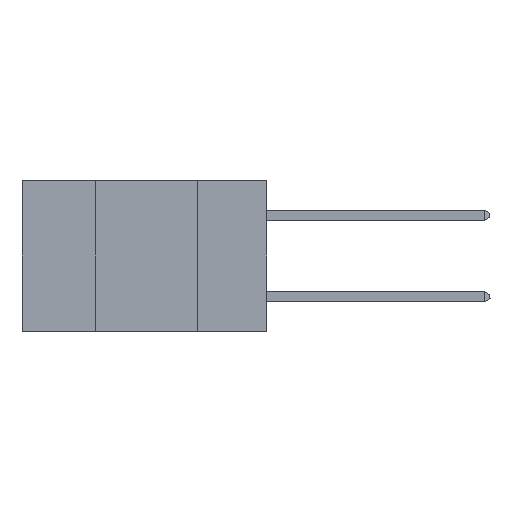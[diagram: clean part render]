
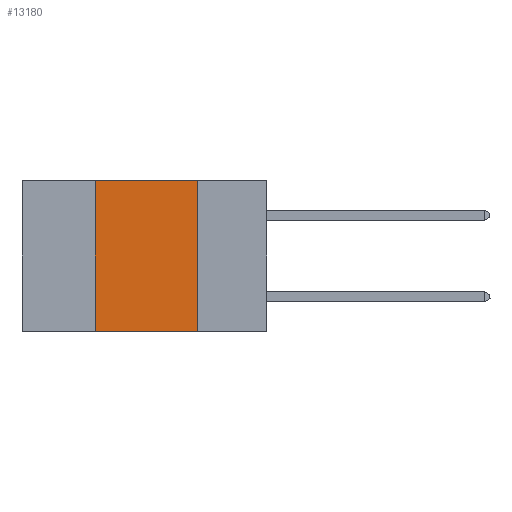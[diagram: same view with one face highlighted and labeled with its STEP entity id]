
A CAD part, left-side view. The second image highlights one B-rep face of the part: STEP entity #13180.
In plain terms, the highlighted planar face has unit normal (-1, 0, 0).
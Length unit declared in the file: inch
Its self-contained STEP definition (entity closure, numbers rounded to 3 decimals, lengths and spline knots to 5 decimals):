
#505 = EDGE_CURVE ( 'NONE', #16563, #8109, #4141, .T. ) ;
#512 = AXIS2_PLACEMENT_3D ( 'NONE', #13867, #15022, #13642 ) ;
#747 = PLANE ( 'NONE',  #512 ) ;
#1017 = EDGE_CURVE ( 'NONE', #11627, #1910, #9396, .T. ) ;
#1866 = ORIENTED_EDGE ( 'NONE', *, *, #1017, .F. ) ;
#1910 = VERTEX_POINT ( 'NONE', #3452 ) ;
#1997 = DIRECTION ( 'NONE',  ( 0., 0., 1. ) ) ;
#2954 = ORIENTED_EDGE ( 'NONE', *, *, #6083, .T. ) ;
#3342 = VECTOR ( 'NONE', #11138, 39.37008 ) ;
#3452 = CARTESIAN_POINT ( 'NONE',  ( 0., 0.17, -0.37 ) ) ;
#4040 = EDGE_LOOP ( 'NONE', ( #1866, #10951, #12915, #2954 ) ) ;
#4141 = LINE ( 'NONE', #8445, #13857 ) ;
#5557 = DIRECTION ( 'NONE',  ( 0., 0., -1. ) ) ;
#6083 = EDGE_CURVE ( 'NONE', #16563, #1910, #7611, .T. ) ;
#7055 = EDGE_CURVE ( 'NONE', #8109, #11627, #14868, .T. ) ;
#7611 = LINE ( 'NONE', #15401, #3342 ) ;
#8109 = VERTEX_POINT ( 'NONE', #9069 ) ;
#8445 = CARTESIAN_POINT ( 'NONE',  ( 0., 0.42, 0. ) ) ;
#9069 = CARTESIAN_POINT ( 'NONE',  ( 0., 0.42, 0. ) ) ;
#9396 = LINE ( 'NONE', #14796, #16338 ) ;
#9911 = FACE_OUTER_BOUND ( 'NONE', #4040, .T. ) ;
#10839 = CARTESIAN_POINT ( 'NONE',  ( 0., 0.17, 0. ) ) ;
#10951 = ORIENTED_EDGE ( 'NONE', *, *, #7055, .F. ) ;
#11138 = DIRECTION ( 'NONE',  ( 0., -1., 0. ) ) ;
#11627 = VERTEX_POINT ( 'NONE', #10839 ) ;
#12032 = DIRECTION ( 'NONE',  ( 0., -1., 0. ) ) ;
#12915 = ORIENTED_EDGE ( 'NONE', *, *, #505, .F. ) ;
#13180 = ADVANCED_FACE ( 'NONE', ( #9911 ), #747, .F. ) ;
#13642 = DIRECTION ( 'NONE',  ( 0., 0., -1. ) ) ;
#13857 = VECTOR ( 'NONE', #1997, 39.37008 ) ;
#13867 = CARTESIAN_POINT ( 'NONE',  ( 0., 0.6, 0. ) ) ;
#14018 = CARTESIAN_POINT ( 'NONE',  ( 0., 0.42, -0.37 ) ) ;
#14796 = CARTESIAN_POINT ( 'NONE',  ( 0., 0.17, 0. ) ) ;
#14868 = LINE ( 'NONE', #16076, #15289 ) ;
#15022 = DIRECTION ( 'NONE',  ( 1., 0., 0. ) ) ;
#15289 = VECTOR ( 'NONE', #12032, 39.37008 ) ;
#15401 = CARTESIAN_POINT ( 'NONE',  ( 0., 0.6, -0.37 ) ) ;
#16076 = CARTESIAN_POINT ( 'NONE',  ( 0., 0.6, 0. ) ) ;
#16338 = VECTOR ( 'NONE', #5557, 39.37008 ) ;
#16563 = VERTEX_POINT ( 'NONE', #14018 ) ;
